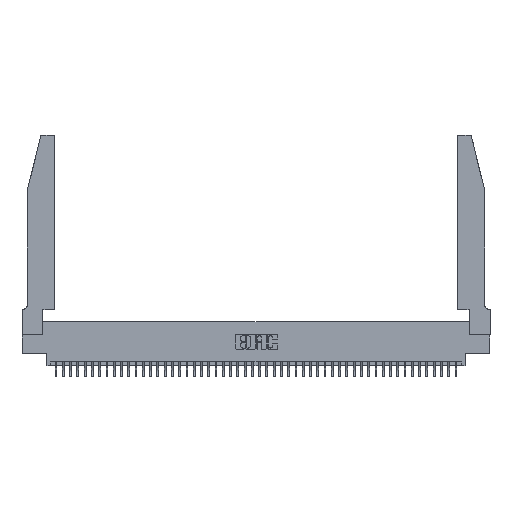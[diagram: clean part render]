
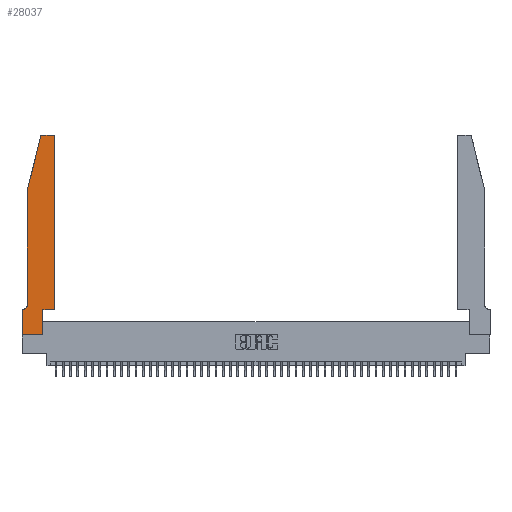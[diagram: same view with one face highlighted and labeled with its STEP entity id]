
A CAD part, top view. The second image highlights one B-rep face of the part: STEP entity #28037.
In plain terms, the highlighted planar face has unit normal (0, 0, 1).
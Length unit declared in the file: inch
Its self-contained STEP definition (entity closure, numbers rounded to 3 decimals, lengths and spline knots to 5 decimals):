
#388 = ORIENTED_EDGE ( 'NONE', *, *, #25807, .T. ) ;
#448 = VECTOR ( 'NONE', #23326, 39.37008 ) ;
#722 = LINE ( 'NONE', #39775, #28751 ) ;
#1381 = CARTESIAN_POINT ( 'NONE',  ( 0., 0., 0.37 ) ) ;
#1477 = DIRECTION ( 'NONE',  ( 0., 1., 0. ) ) ;
#2147 = FACE_OUTER_BOUND ( 'NONE', #29101, .T. ) ;
#2544 = CARTESIAN_POINT ( 'NONE',  ( 0.0755, 0.42, 0.37 ) ) ;
#4520 = EDGE_CURVE ( 'NONE', #43108, #38572, #36973, .T. ) ;
#4724 = ORIENTED_EDGE ( 'NONE', *, *, #4520, .T. ) ;
#5437 = CIRCLE ( 'NONE', #22988, 0.07 ) ;
#5465 = ORIENTED_EDGE ( 'NONE', *, *, #30749, .T. ) ;
#5583 = AXIS2_PLACEMENT_3D ( 'NONE', #18843, #44226, #22502 ) ;
#7329 = CARTESIAN_POINT ( 'NONE',  ( 0.25487, 2.72718, 0.37 ) ) ;
#7664 = VERTEX_POINT ( 'NONE', #34126 ) ;
#7728 = CARTESIAN_POINT ( 'NONE',  ( 0., 0., 0.37 ) ) ;
#8111 = CARTESIAN_POINT ( 'NONE',  ( 0.4505, 2.72, 0.37 ) ) ;
#8260 = VERTEX_POINT ( 'NONE', #37245 ) ;
#8581 = ORIENTED_EDGE ( 'NONE', *, *, #19974, .T. ) ;
#8759 = VERTEX_POINT ( 'NONE', #32951 ) ;
#9210 = DIRECTION ( 'NONE',  ( 0., 0., -1. ) ) ;
#9583 = CARTESIAN_POINT ( 'NONE',  ( 0.284, 2.75, 0.37 ) ) ;
#10664 = DIRECTION ( 'NONE',  ( 0., 0., 1. ) ) ;
#11094 = ORIENTED_EDGE ( 'NONE', *, *, #28354, .T. ) ;
#11564 = VECTOR ( 'NONE', #45244, 39.37008 ) ;
#12316 = EDGE_CURVE ( 'NONE', #38572, #8759, #41712, .T. ) ;
#12509 = CARTESIAN_POINT ( 'NONE',  ( 0.0755, 0.35, 0.37 ) ) ;
#12587 = CARTESIAN_POINT ( 'NONE',  ( 0.2865, 0.35, 0.37 ) ) ;
#12629 = ORIENTED_EDGE ( 'NONE', *, *, #12653, .T. ) ;
#12653 = EDGE_CURVE ( 'NONE', #25128, #8260, #38829, .T. ) ;
#13392 = VECTOR ( 'NONE', #27429, 39.37008 ) ;
#14882 = ORIENTED_EDGE ( 'NONE', *, *, #40230, .T. ) ;
#15047 = ORIENTED_EDGE ( 'NONE', *, *, #43308, .T. ) ;
#15124 = VERTEX_POINT ( 'NONE', #44552 ) ;
#15366 = CIRCLE ( 'NONE', #31617, 0.03 ) ;
#16037 = DIRECTION ( 'NONE',  ( -0.239, -0.971, 0. ) ) ;
#17701 = CIRCLE ( 'NONE', #5583, 0.03 ) ;
#17823 = VERTEX_POINT ( 'NONE', #28523 ) ;
#18188 = DIRECTION ( 'NONE',  ( 0., 1., 0. ) ) ;
#18843 = CARTESIAN_POINT ( 'NONE',  ( 0.284, 2.72, 0.37 ) ) ;
#19598 = ORIENTED_EDGE ( 'NONE', *, *, #39905, .T. ) ;
#19974 = EDGE_CURVE ( 'NONE', #46375, #25128, #17701, .T. ) ;
#20025 = DIRECTION ( 'NONE',  ( 1., 0., 0. ) ) ;
#20503 = EDGE_CURVE ( 'NONE', #35083, #7664, #15366, .T. ) ;
#20748 = VECTOR ( 'NONE', #18188, 39.37008 ) ;
#21259 = LINE ( 'NONE', #12509, #11564 ) ;
#22502 = DIRECTION ( 'NONE',  ( 1., 0., 0. ) ) ;
#22961 = VECTOR ( 'NONE', #16037, 39.37008 ) ;
#22988 = AXIS2_PLACEMENT_3D ( 'NONE', #31031, #9210, #34688 ) ;
#23326 = DIRECTION ( 'NONE',  ( 1., 0., 0. ) ) ;
#23509 = PLANE ( 'NONE',  #38717 ) ;
#25128 = VERTEX_POINT ( 'NONE', #7329 ) ;
#25807 = EDGE_CURVE ( 'NONE', #15124, #35083, #38891, .T. ) ;
#26304 = VERTEX_POINT ( 'NONE', #2544 ) ;
#27308 = LINE ( 'NONE', #39659, #45462 ) ;
#27429 = DIRECTION ( 'NONE',  ( 0., -1., 0. ) ) ;
#28037 = ADVANCED_FACE ( 'NONE', ( #2147 ), #23509, .T. ) ;
#28354 = EDGE_CURVE ( 'NONE', #17823, #43108, #27308, .T. ) ;
#28523 = CARTESIAN_POINT ( 'NONE',  ( 0., 0.35, 0.37 ) ) ;
#28751 = VECTOR ( 'NONE', #28847, 39.37008 ) ;
#28847 = DIRECTION ( 'NONE',  ( -1., 0., 0. ) ) ;
#28879 = CARTESIAN_POINT ( 'NONE',  ( 0.2865, 0., 0.37 ) ) ;
#29101 = EDGE_LOOP ( 'NONE', ( #14882, #8581, #12629, #19598, #34406, #15047, #11094, #4724, #37947, #5465, #388, #40323 ) ) ;
#30749 = EDGE_CURVE ( 'NONE', #8759, #15124, #33853, .T. ) ;
#30835 = CARTESIAN_POINT ( 'NONE',  ( 0., 0.35, 0.37 ) ) ;
#31031 = CARTESIAN_POINT ( 'NONE',  ( 0.0055, 0.42, 0.37 ) ) ;
#31092 = CARTESIAN_POINT ( 'NONE',  ( 0.0755, 2., 0.37 ) ) ;
#31583 = VERTEX_POINT ( 'NONE', #37702 ) ;
#31617 = AXIS2_PLACEMENT_3D ( 'NONE', #32475, #10664, #36106 ) ;
#32094 = VECTOR ( 'NONE', #1477, 39.37008 ) ;
#32475 = CARTESIAN_POINT ( 'NONE',  ( 0.4205, 2.72, 0.37 ) ) ;
#32588 = CARTESIAN_POINT ( 'NONE',  ( 0.4505, 0.35, 0.37 ) ) ;
#32775 = LINE ( 'NONE', #31092, #13392 ) ;
#32951 = CARTESIAN_POINT ( 'NONE',  ( 0.2865, 0.35, 0.37 ) ) ;
#33853 = LINE ( 'NONE', #32588, #34989 ) ;
#34126 = CARTESIAN_POINT ( 'NONE',  ( 0.4205, 2.75, 0.37 ) ) ;
#34406 = ORIENTED_EDGE ( 'NONE', *, *, #47023, .T. ) ;
#34688 = DIRECTION ( 'NONE',  ( -1., 0., 0. ) ) ;
#34989 = VECTOR ( 'NONE', #47159, 39.37008 ) ;
#35083 = VERTEX_POINT ( 'NONE', #8111 ) ;
#36106 = DIRECTION ( 'NONE',  ( 1., 0., 0. ) ) ;
#36973 = LINE ( 'NONE', #1381, #448 ) ;
#37245 = CARTESIAN_POINT ( 'NONE',  ( 0.0755, 2., 0.37 ) ) ;
#37702 = CARTESIAN_POINT ( 'NONE',  ( 0.0055, 0.35, 0.37 ) ) ;
#37778 = CARTESIAN_POINT ( 'NONE',  ( 0.0755, 2., 0.37 ) ) ;
#37947 = ORIENTED_EDGE ( 'NONE', *, *, #12316, .T. ) ;
#38572 = VERTEX_POINT ( 'NONE', #28879 ) ;
#38717 = AXIS2_PLACEMENT_3D ( 'NONE', #30835, #41746, #20025 ) ;
#38829 = LINE ( 'NONE', #37778, #22961 ) ;
#38891 = LINE ( 'NONE', #43562, #20748 ) ;
#39659 = CARTESIAN_POINT ( 'NONE',  ( 0., 0., 0.37 ) ) ;
#39775 = CARTESIAN_POINT ( 'NONE',  ( 0.2605, 2.75, 0.37 ) ) ;
#39905 = EDGE_CURVE ( 'NONE', #8260, #26304, #32775, .T. ) ;
#40230 = EDGE_CURVE ( 'NONE', #7664, #46375, #722, .T. ) ;
#40323 = ORIENTED_EDGE ( 'NONE', *, *, #20503, .T. ) ;
#41712 = LINE ( 'NONE', #12587, #32094 ) ;
#41746 = DIRECTION ( 'NONE',  ( 0., 0., 1. ) ) ;
#43108 = VERTEX_POINT ( 'NONE', #7728 ) ;
#43307 = DIRECTION ( 'NONE',  ( 0., -1., 0. ) ) ;
#43308 = EDGE_CURVE ( 'NONE', #31583, #17823, #21259, .T. ) ;
#43562 = CARTESIAN_POINT ( 'NONE',  ( 0.4505, 0.35, 0.37 ) ) ;
#44226 = DIRECTION ( 'NONE',  ( 0., 0., 1. ) ) ;
#44552 = CARTESIAN_POINT ( 'NONE',  ( 0.4505, 0.35, 0.37 ) ) ;
#45244 = DIRECTION ( 'NONE',  ( -1., 0., 0. ) ) ;
#45462 = VECTOR ( 'NONE', #43307, 39.37008 ) ;
#46375 = VERTEX_POINT ( 'NONE', #9583 ) ;
#47023 = EDGE_CURVE ( 'NONE', #26304, #31583, #5437, .T. ) ;
#47159 = DIRECTION ( 'NONE',  ( 1., 0., 0. ) ) ;
